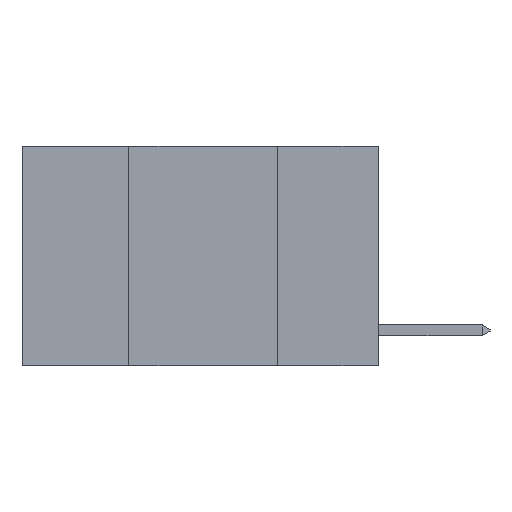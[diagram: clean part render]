
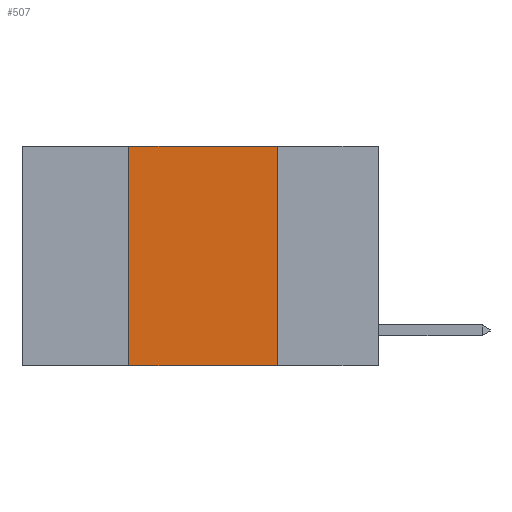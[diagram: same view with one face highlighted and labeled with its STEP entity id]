
A CAD part, left-side view. The second image highlights one B-rep face of the part: STEP entity #507.
In plain terms, the highlighted planar face has unit normal (-1, 0, 0).
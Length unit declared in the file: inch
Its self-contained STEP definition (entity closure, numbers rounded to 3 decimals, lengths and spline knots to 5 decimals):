
#492 = CARTESIAN_POINT ( 'NONE',  ( 0., 0.42, -0.37 ) ) ;
#507 = ADVANCED_FACE ( 'NONE', ( #2828 ), #3669, .F. ) ;
#611 = VECTOR ( 'NONE', #2094, 39.37008 ) ;
#1111 = ORIENTED_EDGE ( 'NONE', *, *, #3797, .F. ) ;
#1300 = CARTESIAN_POINT ( 'NONE',  ( 0., 0.6, -0.37 ) ) ;
#1439 = CARTESIAN_POINT ( 'NONE',  ( 0., 0.6, 0. ) ) ;
#1574 = CARTESIAN_POINT ( 'NONE',  ( 0., 0.17, 0. ) ) ;
#1607 = DIRECTION ( 'NONE',  ( 0., 0., -1. ) ) ;
#1774 = LINE ( 'NONE', #1574, #9730 ) ;
#1892 = CARTESIAN_POINT ( 'NONE',  ( 0., 0.42, 0. ) ) ;
#2094 = DIRECTION ( 'NONE',  ( 0., -1., 0. ) ) ;
#2144 = ORIENTED_EDGE ( 'NONE', *, *, #2686, .T. ) ;
#2686 = EDGE_CURVE ( 'NONE', #5236, #3980, #2777, .T. ) ;
#2777 = LINE ( 'NONE', #1300, #611 ) ;
#2795 = LINE ( 'NONE', #7666, #4845 ) ;
#2828 = FACE_OUTER_BOUND ( 'NONE', #9742, .T. ) ;
#2928 = EDGE_CURVE ( 'NONE', #9305, #3980, #1774, .T. ) ;
#2932 = CARTESIAN_POINT ( 'NONE',  ( 0., 0.17, -0.37 ) ) ;
#3666 = DIRECTION ( 'NONE',  ( 1., 0., 0. ) ) ;
#3669 = PLANE ( 'NONE',  #8738 ) ;
#3797 = EDGE_CURVE ( 'NONE', #5236, #7686, #4786, .T. ) ;
#3810 = DIRECTION ( 'NONE',  ( 0., -1., 0. ) ) ;
#3980 = VERTEX_POINT ( 'NONE', #2932 ) ;
#4549 = VECTOR ( 'NONE', #6555, 39.37008 ) ;
#4786 = LINE ( 'NONE', #1892, #4549 ) ;
#4845 = VECTOR ( 'NONE', #3810, 39.37008 ) ;
#5236 = VERTEX_POINT ( 'NONE', #492 ) ;
#5261 = ORIENTED_EDGE ( 'NONE', *, *, #2928, .F. ) ;
#5797 = CARTESIAN_POINT ( 'NONE',  ( 0., 0.17, 0. ) ) ;
#6555 = DIRECTION ( 'NONE',  ( 0., 0., 1. ) ) ;
#7329 = EDGE_CURVE ( 'NONE', #7686, #9305, #2795, .T. ) ;
#7666 = CARTESIAN_POINT ( 'NONE',  ( 0., 0.6, 0. ) ) ;
#7686 = VERTEX_POINT ( 'NONE', #8986 ) ;
#8148 = ORIENTED_EDGE ( 'NONE', *, *, #7329, .F. ) ;
#8738 = AXIS2_PLACEMENT_3D ( 'NONE', #1439, #3666, #10025 ) ;
#8986 = CARTESIAN_POINT ( 'NONE',  ( 0., 0.42, 0. ) ) ;
#9305 = VERTEX_POINT ( 'NONE', #5797 ) ;
#9730 = VECTOR ( 'NONE', #1607, 39.37008 ) ;
#9742 = EDGE_LOOP ( 'NONE', ( #5261, #8148, #1111, #2144 ) ) ;
#10025 = DIRECTION ( 'NONE',  ( 0., 0., -1. ) ) ;
